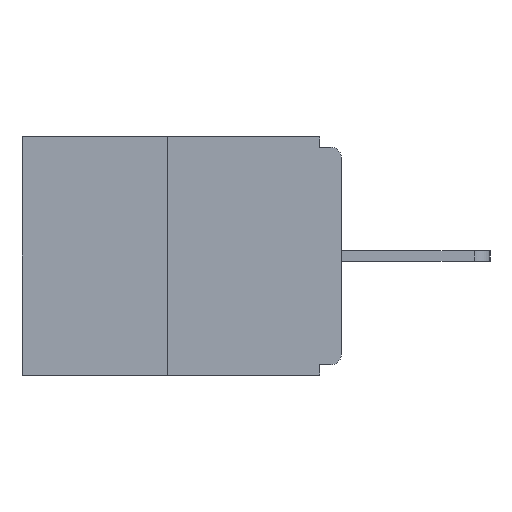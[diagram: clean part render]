
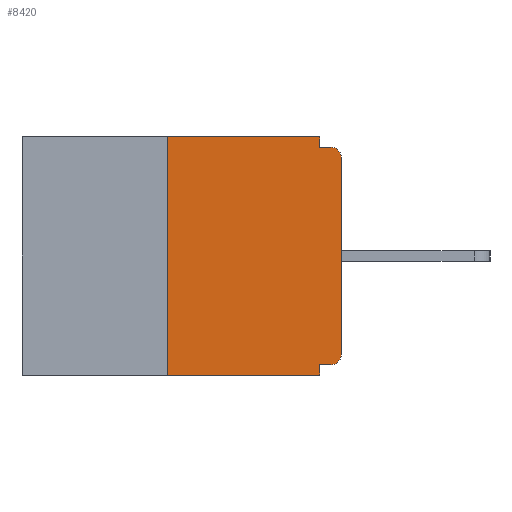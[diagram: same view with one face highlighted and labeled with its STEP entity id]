
A CAD part, left-side view. The second image highlights one B-rep face of the part: STEP entity #8420.
In plain terms, the highlighted planar face has unit normal (-1, 0, 0).
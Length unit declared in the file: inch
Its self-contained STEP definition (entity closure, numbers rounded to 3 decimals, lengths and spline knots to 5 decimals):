
#144 = DIRECTION ( 'NONE',  ( 0., -1., 0. ) ) ;
#316 = CARTESIAN_POINT ( 'NONE',  ( 0., 0.031, -0.343 ) ) ;
#404 = ORIENTED_EDGE ( 'NONE', *, *, #6619, .F. ) ;
#649 = AXIS2_PLACEMENT_3D ( 'NONE', #18429, #8976, #11174 ) ;
#753 = VERTEX_POINT ( 'NONE', #11207 ) ;
#790 = VECTOR ( 'NONE', #11289, 39.37008 ) ;
#1181 = CARTESIAN_POINT ( 'NONE',  ( 0., 0.25, -0.343 ) ) ;
#2192 = ORIENTED_EDGE ( 'NONE', *, *, #9626, .F. ) ;
#2296 = VECTOR ( 'NONE', #11639, 39.37008 ) ;
#2904 = VERTEX_POINT ( 'NONE', #8199 ) ;
#2909 = ORIENTED_EDGE ( 'NONE', *, *, #22940, .F. ) ;
#3085 = LINE ( 'NONE', #10554, #6582 ) ;
#3597 = AXIS2_PLACEMENT_3D ( 'NONE', #14079, #12245, #19763 ) ;
#3687 = FACE_OUTER_BOUND ( 'NONE', #21922, .T. ) ;
#4226 = DIRECTION ( 'NONE',  ( -1., 0., 0. ) ) ;
#4381 = DIRECTION ( 'NONE',  ( 0., -1., 0. ) ) ;
#4400 = ORIENTED_EDGE ( 'NONE', *, *, #8373, .F. ) ;
#5033 = VERTEX_POINT ( 'NONE', #16847 ) ;
#5945 = VECTOR ( 'NONE', #4381, 39.37008 ) ;
#5998 = VERTEX_POINT ( 'NONE', #11975 ) ;
#6582 = VECTOR ( 'NONE', #18049, 39.37008 ) ;
#6619 = EDGE_CURVE ( 'NONE', #2904, #5033, #15219, .T. ) ;
#6893 = CARTESIAN_POINT ( 'NONE',  ( 0., 0., -0.313 ) ) ;
#6942 = DIRECTION ( 'NONE',  ( 0., 0., 1. ) ) ;
#7133 = LINE ( 'NONE', #13003, #15891 ) ;
#7357 = VECTOR ( 'NONE', #6942, 39.37008 ) ;
#7784 = DIRECTION ( 'NONE',  ( 0., 0., -1. ) ) ;
#7993 = CARTESIAN_POINT ( 'NONE',  ( 0., 0., -0.03 ) ) ;
#8199 = CARTESIAN_POINT ( 'NONE',  ( 0., 0.031, -0.015 ) ) ;
#8208 = AXIS2_PLACEMENT_3D ( 'NONE', #13535, #4226, #16995 ) ;
#8373 = EDGE_CURVE ( 'NONE', #5998, #9604, #7133, .T. ) ;
#8420 = ADVANCED_FACE ( 'NONE', ( #3687 ), #13249, .F. ) ;
#8884 = ORIENTED_EDGE ( 'NONE', *, *, #15584, .T. ) ;
#8976 = DIRECTION ( 'NONE',  ( 1., 0., 0. ) ) ;
#9604 = VERTEX_POINT ( 'NONE', #12881 ) ;
#9626 = EDGE_CURVE ( 'NONE', #21622, #5998, #22277, .T. ) ;
#9796 = CARTESIAN_POINT ( 'NONE',  ( 0., 0., -0.328 ) ) ;
#10554 = CARTESIAN_POINT ( 'NONE',  ( 0., 0.031, 0. ) ) ;
#11174 = DIRECTION ( 'NONE',  ( 0., 0., -1. ) ) ;
#11207 = CARTESIAN_POINT ( 'NONE',  ( 0., 0.031, -0.343 ) ) ;
#11289 = DIRECTION ( 'NONE',  ( 0., -1., 0. ) ) ;
#11546 = ORIENTED_EDGE ( 'NONE', *, *, #23029, .T. ) ;
#11639 = DIRECTION ( 'NONE',  ( 0., 1., 0. ) ) ;
#11975 = CARTESIAN_POINT ( 'NONE',  ( 0., 0.25, 0. ) ) ;
#12245 = DIRECTION ( 'NONE',  ( -1., 0., 0. ) ) ;
#12881 = CARTESIAN_POINT ( 'NONE',  ( 0., 0.031, 0. ) ) ;
#13003 = CARTESIAN_POINT ( 'NONE',  ( 0., 0.46, 0. ) ) ;
#13249 = PLANE ( 'NONE',  #649 ) ;
#13325 = CARTESIAN_POINT ( 'NONE',  ( 0., 0.46, -0.343 ) ) ;
#13535 = CARTESIAN_POINT ( 'NONE',  ( 0., 0.015, -0.313 ) ) ;
#14079 = CARTESIAN_POINT ( 'NONE',  ( 0., 0.015, -0.03 ) ) ;
#14231 = EDGE_CURVE ( 'NONE', #23719, #5033, #22851, .T. ) ;
#14494 = ORIENTED_EDGE ( 'NONE', *, *, #14809, .F. ) ;
#14809 = EDGE_CURVE ( 'NONE', #16267, #753, #18723, .T. ) ;
#15219 = LINE ( 'NONE', #18914, #790 ) ;
#15256 = CIRCLE ( 'NONE', #8208, 0.015 ) ;
#15314 = LINE ( 'NONE', #13325, #5945 ) ;
#15584 = EDGE_CURVE ( 'NONE', #21622, #753, #15314, .T. ) ;
#15891 = VECTOR ( 'NONE', #144, 39.37008 ) ;
#16267 = VERTEX_POINT ( 'NONE', #21162 ) ;
#16504 = VECTOR ( 'NONE', #7784, 39.37008 ) ;
#16836 = DIRECTION ( 'NONE',  ( 0., 0., 1. ) ) ;
#16847 = CARTESIAN_POINT ( 'NONE',  ( 0., 0.015, -0.015 ) ) ;
#16910 = ORIENTED_EDGE ( 'NONE', *, *, #22711, .F. ) ;
#16995 = DIRECTION ( 'NONE',  ( 0., 0., -1. ) ) ;
#17647 = LINE ( 'NONE', #9796, #2296 ) ;
#18049 = DIRECTION ( 'NONE',  ( 0., 0., -1. ) ) ;
#18429 = CARTESIAN_POINT ( 'NONE',  ( 0., 0.46, 0. ) ) ;
#18555 = CARTESIAN_POINT ( 'NONE',  ( 0., 0.25, 0. ) ) ;
#18723 = LINE ( 'NONE', #316, #16504 ) ;
#18780 = VERTEX_POINT ( 'NONE', #6893 ) ;
#18914 = CARTESIAN_POINT ( 'NONE',  ( 0., 0., -0.015 ) ) ;
#19443 = CARTESIAN_POINT ( 'NONE',  ( 0., 0.015, -0.328 ) ) ;
#19717 = ORIENTED_EDGE ( 'NONE', *, *, #23211, .T. ) ;
#19763 = DIRECTION ( 'NONE',  ( 0., 0., -1. ) ) ;
#20451 = CARTESIAN_POINT ( 'NONE',  ( 0., 0., 0. ) ) ;
#20748 = VERTEX_POINT ( 'NONE', #19443 ) ;
#21162 = CARTESIAN_POINT ( 'NONE',  ( 0., 0.031, -0.328 ) ) ;
#21622 = VERTEX_POINT ( 'NONE', #1181 ) ;
#21922 = EDGE_LOOP ( 'NONE', ( #4400, #2192, #8884, #14494, #2909, #19717, #11546, #22515, #404, #16910 ) ) ;
#22140 = VECTOR ( 'NONE', #16836, 39.37008 ) ;
#22277 = LINE ( 'NONE', #18555, #22140 ) ;
#22515 = ORIENTED_EDGE ( 'NONE', *, *, #14231, .T. ) ;
#22711 = EDGE_CURVE ( 'NONE', #9604, #2904, #3085, .T. ) ;
#22851 = CIRCLE ( 'NONE', #3597, 0.015 ) ;
#22940 = EDGE_CURVE ( 'NONE', #20748, #16267, #17647, .T. ) ;
#23029 = EDGE_CURVE ( 'NONE', #18780, #23719, #24142, .T. ) ;
#23211 = EDGE_CURVE ( 'NONE', #20748, #18780, #15256, .T. ) ;
#23719 = VERTEX_POINT ( 'NONE', #7993 ) ;
#24142 = LINE ( 'NONE', #20451, #7357 ) ;
